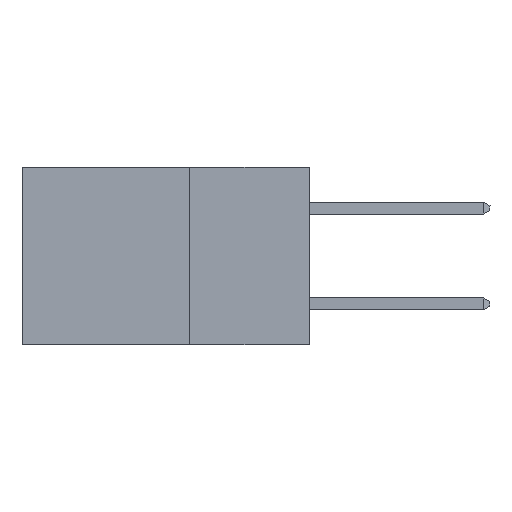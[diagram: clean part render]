
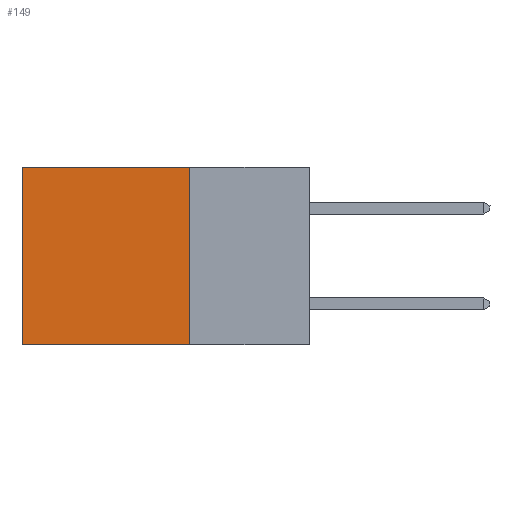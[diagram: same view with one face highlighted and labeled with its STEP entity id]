
A CAD part, left-side view. The second image highlights one B-rep face of the part: STEP entity #149.
In plain terms, the highlighted planar face has unit normal (-1, 0, 0).
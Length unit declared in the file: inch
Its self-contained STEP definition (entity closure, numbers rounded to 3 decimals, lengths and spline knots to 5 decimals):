
#33 = VERTEX_POINT ( 'NONE', #1855 ) ;
#149 = ADVANCED_FACE ( 'NONE', ( #1564 ), #7243, .F. ) ;
#155 = LINE ( 'NONE', #11941, #13229 ) ;
#266 = CARTESIAN_POINT ( 'NONE',  ( 0.2875, 0.6, -0.37 ) ) ;
#442 = VECTOR ( 'NONE', #7321, 39.37008 ) ;
#1140 = ORIENTED_EDGE ( 'NONE', *, *, #14300, .F. ) ;
#1142 = EDGE_CURVE ( 'NONE', #5053, #33, #3807, .T. ) ;
#1564 = FACE_OUTER_BOUND ( 'NONE', #8545, .T. ) ;
#1566 = ORIENTED_EDGE ( 'NONE', *, *, #10800, .F. ) ;
#1782 = ORIENTED_EDGE ( 'NONE', *, *, #1142, .T. ) ;
#1855 = CARTESIAN_POINT ( 'NONE',  ( 0.2875, 0.6, 0. ) ) ;
#2767 = DIRECTION ( 'NONE',  ( 1., 0., 0. ) ) ;
#2982 = CARTESIAN_POINT ( 'NONE',  ( 0.2875, 0.25, -0.37 ) ) ;
#3593 = VERTEX_POINT ( 'NONE', #266 ) ;
#3718 = VERTEX_POINT ( 'NONE', #15021 ) ;
#3807 = LINE ( 'NONE', #12588, #13701 ) ;
#4541 = DIRECTION ( 'NONE',  ( 0., 0., -1. ) ) ;
#5053 = VERTEX_POINT ( 'NONE', #6001 ) ;
#5522 = VECTOR ( 'NONE', #5624, 39.37008 ) ;
#5624 = DIRECTION ( 'NONE',  ( 0., 1., 0. ) ) ;
#5919 = ORIENTED_EDGE ( 'NONE', *, *, #6949, .T. ) ;
#6001 = CARTESIAN_POINT ( 'NONE',  ( 0.2875, 0.25, 0. ) ) ;
#6118 = CARTESIAN_POINT ( 'NONE',  ( 0.2875, 0.25, 0. ) ) ;
#6231 = DIRECTION ( 'NONE',  ( 0., 0., -1. ) ) ;
#6949 = EDGE_CURVE ( 'NONE', #33, #3593, #155, .T. ) ;
#7243 = PLANE ( 'NONE',  #14718 ) ;
#7321 = DIRECTION ( 'NONE',  ( 0., 0., -1. ) ) ;
#8545 = EDGE_LOOP ( 'NONE', ( #5919, #1140, #1566, #1782 ) ) ;
#9269 = CARTESIAN_POINT ( 'NONE',  ( 0.2875, 0.25, 0. ) ) ;
#10583 = LINE ( 'NONE', #6118, #442 ) ;
#10800 = EDGE_CURVE ( 'NONE', #5053, #3718, #10583, .T. ) ;
#11941 = CARTESIAN_POINT ( 'NONE',  ( 0.2875, 0.6, 0. ) ) ;
#12588 = CARTESIAN_POINT ( 'NONE',  ( 0.2875, 0.25, 0. ) ) ;
#13062 = DIRECTION ( 'NONE',  ( 0., 1., 0. ) ) ;
#13229 = VECTOR ( 'NONE', #4541, 39.37008 ) ;
#13701 = VECTOR ( 'NONE', #13062, 39.37008 ) ;
#14300 = EDGE_CURVE ( 'NONE', #3718, #3593, #15160, .T. ) ;
#14718 = AXIS2_PLACEMENT_3D ( 'NONE', #9269, #2767, #6231 ) ;
#15021 = CARTESIAN_POINT ( 'NONE',  ( 0.2875, 0.25, -0.37 ) ) ;
#15160 = LINE ( 'NONE', #2982, #5522 ) ;
